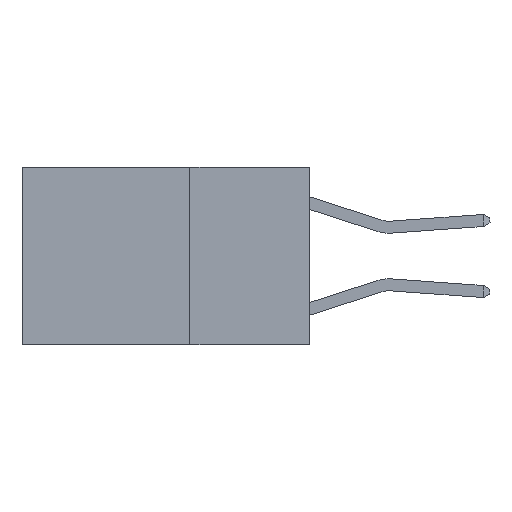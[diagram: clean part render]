
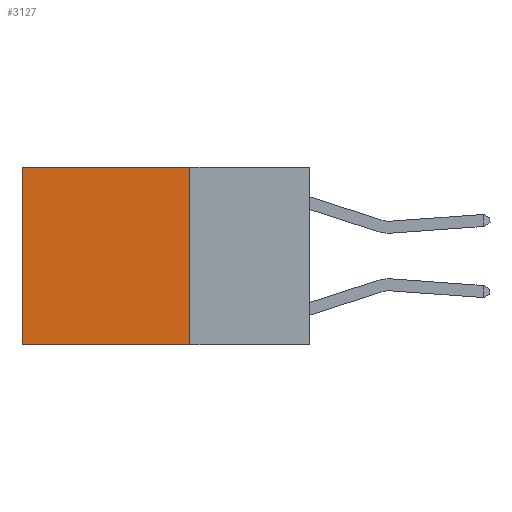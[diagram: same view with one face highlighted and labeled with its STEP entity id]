
A CAD part, left-side view. The second image highlights one B-rep face of the part: STEP entity #3127.
In plain terms, the highlighted planar face has unit normal (-1, 0, 0).
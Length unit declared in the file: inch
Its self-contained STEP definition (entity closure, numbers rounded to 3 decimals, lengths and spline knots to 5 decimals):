
#425 = AXIS2_PLACEMENT_3D ( 'NONE', #9741, #2832, #9848 ) ;
#474 = ORIENTED_EDGE ( 'NONE', *, *, #7734, .F. ) ;
#578 = DIRECTION ( 'NONE',  ( 0., 1., 0. ) ) ;
#797 = VERTEX_POINT ( 'NONE', #1949 ) ;
#809 = VECTOR ( 'NONE', #578, 39.37008 ) ;
#876 = EDGE_CURVE ( 'NONE', #5145, #10193, #7861, .T. ) ;
#1573 = EDGE_CURVE ( 'NONE', #797, #7869, #9560, .T. ) ;
#1949 = CARTESIAN_POINT ( 'NONE',  ( 0.2625, 0.6, 0. ) ) ;
#2221 = CARTESIAN_POINT ( 'NONE',  ( 0.2625, 0.25, -0.37 ) ) ;
#2359 = ORIENTED_EDGE ( 'NONE', *, *, #1573, .T. ) ;
#2457 = VECTOR ( 'NONE', #9041, 39.37008 ) ;
#2825 = VECTOR ( 'NONE', #6144, 39.37008 ) ;
#2832 = DIRECTION ( 'NONE',  ( 1., 0., 0. ) ) ;
#3127 = ADVANCED_FACE ( 'NONE', ( #7864 ), #4532, .F. ) ;
#3174 = LINE ( 'NONE', #2221, #809 ) ;
#3667 = CARTESIAN_POINT ( 'NONE',  ( 0.2625, 0.25, 0. ) ) ;
#4292 = VECTOR ( 'NONE', #9214, 39.37008 ) ;
#4532 = PLANE ( 'NONE',  #425 ) ;
#5145 = VERTEX_POINT ( 'NONE', #5642 ) ;
#5360 = EDGE_CURVE ( 'NONE', #5145, #797, #9857, .T. ) ;
#5444 = EDGE_LOOP ( 'NONE', ( #2359, #474, #11123, #8234 ) ) ;
#5567 = CARTESIAN_POINT ( 'NONE',  ( 0.2625, 0.25, -0.37 ) ) ;
#5642 = CARTESIAN_POINT ( 'NONE',  ( 0.2625, 0.25, 0. ) ) ;
#6144 = DIRECTION ( 'NONE',  ( 0., 1., 0. ) ) ;
#7734 = EDGE_CURVE ( 'NONE', #10193, #7869, #3174, .T. ) ;
#7861 = LINE ( 'NONE', #3667, #2457 ) ;
#7864 = FACE_OUTER_BOUND ( 'NONE', #5444, .T. ) ;
#7869 = VERTEX_POINT ( 'NONE', #9701 ) ;
#8234 = ORIENTED_EDGE ( 'NONE', *, *, #5360, .T. ) ;
#9041 = DIRECTION ( 'NONE',  ( 0., 0., -1. ) ) ;
#9214 = DIRECTION ( 'NONE',  ( 0., 0., -1. ) ) ;
#9318 = CARTESIAN_POINT ( 'NONE',  ( 0.2625, 0.6, 0. ) ) ;
#9560 = LINE ( 'NONE', #9318, #4292 ) ;
#9701 = CARTESIAN_POINT ( 'NONE',  ( 0.2625, 0.6, -0.37 ) ) ;
#9741 = CARTESIAN_POINT ( 'NONE',  ( 0.2625, 0.25, 0. ) ) ;
#9848 = DIRECTION ( 'NONE',  ( 0., 0., -1. ) ) ;
#9857 = LINE ( 'NONE', #11144, #2825 ) ;
#10193 = VERTEX_POINT ( 'NONE', #5567 ) ;
#11123 = ORIENTED_EDGE ( 'NONE', *, *, #876, .F. ) ;
#11144 = CARTESIAN_POINT ( 'NONE',  ( 0.2625, 0.25, 0. ) ) ;
